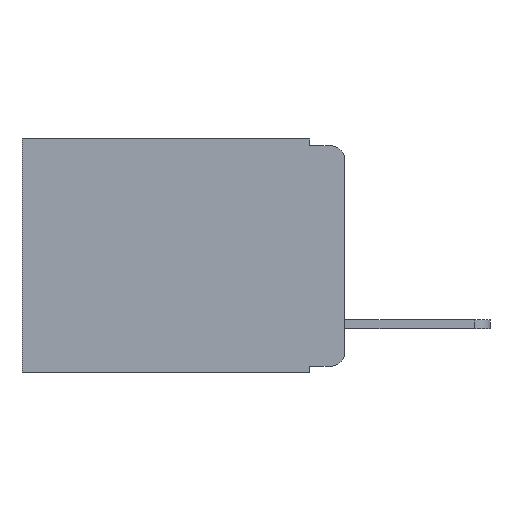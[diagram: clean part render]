
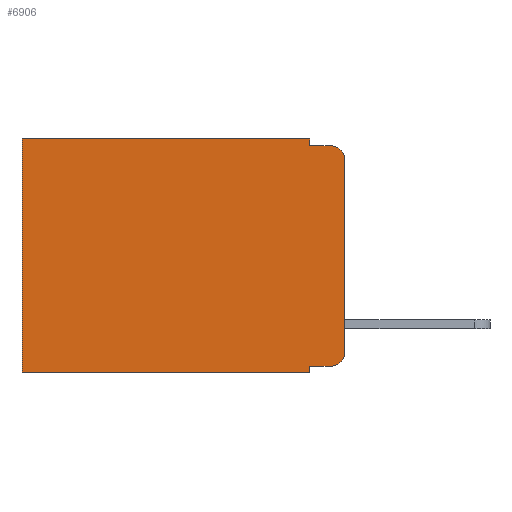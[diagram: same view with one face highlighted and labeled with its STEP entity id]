
A CAD part, left-side view. The second image highlights one B-rep face of the part: STEP entity #6906.
In plain terms, the highlighted planar face has unit normal (-1, 0, 0).
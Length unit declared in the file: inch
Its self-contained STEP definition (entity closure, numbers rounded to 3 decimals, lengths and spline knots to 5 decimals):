
#186 = DIRECTION ( 'NONE',  ( -1., 0., 0. ) ) ;
#322 = VERTEX_POINT ( 'NONE', #6644 ) ;
#1063 = ORIENTED_EDGE ( 'NONE', *, *, #12610, .F. ) ;
#1539 = ORIENTED_EDGE ( 'NONE', *, *, #17304, .T. ) ;
#1707 = PLANE ( 'NONE',  #15708 ) ;
#1716 = AXIS2_PLACEMENT_3D ( 'NONE', #11540, #2862, #12925 ) ;
#1764 = CARTESIAN_POINT ( 'NONE',  ( 0.298, 0.051, -0.333 ) ) ;
#1904 = VERTEX_POINT ( 'NONE', #14746 ) ;
#2031 = ORIENTED_EDGE ( 'NONE', *, *, #14384, .F. ) ;
#2276 = VERTEX_POINT ( 'NONE', #9889 ) ;
#2442 = CARTESIAN_POINT ( 'NONE',  ( 0.298, 0.02, -0.01 ) ) ;
#2471 = ORIENTED_EDGE ( 'NONE', *, *, #9795, .F. ) ;
#2862 = DIRECTION ( 'NONE',  ( -1., 0., 0. ) ) ;
#3031 = DIRECTION ( 'NONE',  ( 0., 1., 0. ) ) ;
#3351 = CARTESIAN_POINT ( 'NONE',  ( 0.298, 0.02, -0.333 ) ) ;
#3567 = EDGE_CURVE ( 'NONE', #14981, #322, #12521, .T. ) ;
#3623 = ORIENTED_EDGE ( 'NONE', *, *, #11748, .F. ) ;
#4083 = CARTESIAN_POINT ( 'NONE',  ( 0.298, 0.051, 0. ) ) ;
#4109 = ORIENTED_EDGE ( 'NONE', *, *, #16272, .T. ) ;
#4199 = LINE ( 'NONE', #12186, #15170 ) ;
#4616 = LINE ( 'NONE', #12272, #8509 ) ;
#4727 = AXIS2_PLACEMENT_3D ( 'NONE', #9014, #186, #10432 ) ;
#5464 = EDGE_CURVE ( 'NONE', #13408, #322, #7833, .T. ) ;
#5963 = EDGE_CURVE ( 'NONE', #9986, #2276, #11130, .T. ) ;
#5988 = CARTESIAN_POINT ( 'NONE',  ( 0.298, 0., -0.03 ) ) ;
#6644 = CARTESIAN_POINT ( 'NONE',  ( 0.298, 0., -0.313 ) ) ;
#6906 = ADVANCED_FACE ( 'NONE', ( #13041 ), #1707, .F. ) ;
#7362 = ORIENTED_EDGE ( 'NONE', *, *, #5464, .T. ) ;
#7469 = CARTESIAN_POINT ( 'NONE',  ( 0.298, 0.051, 0. ) ) ;
#7648 = CARTESIAN_POINT ( 'NONE',  ( 0.298, 0., 0. ) ) ;
#7833 = CIRCLE ( 'NONE', #1716, 0.02 ) ;
#8217 = VERTEX_POINT ( 'NONE', #1764 ) ;
#8253 = LINE ( 'NONE', #7469, #11129 ) ;
#8509 = VECTOR ( 'NONE', #13670, 39.37008 ) ;
#8649 = ORIENTED_EDGE ( 'NONE', *, *, #3567, .F. ) ;
#9014 = CARTESIAN_POINT ( 'NONE',  ( 0.298, 0.02, -0.03 ) ) ;
#9064 = DIRECTION ( 'NONE',  ( 0., 0., -1. ) ) ;
#9400 = LINE ( 'NONE', #12596, #16417 ) ;
#9449 = LINE ( 'NONE', #13087, #17327 ) ;
#9788 = CARTESIAN_POINT ( 'NONE',  ( 0.298, 0.473, 0. ) ) ;
#9795 = EDGE_CURVE ( 'NONE', #15896, #11441, #17621, .T. ) ;
#9889 = CARTESIAN_POINT ( 'NONE',  ( 0.298, 0.473, -0.343 ) ) ;
#9986 = VERTEX_POINT ( 'NONE', #15990 ) ;
#10327 = VERTEX_POINT ( 'NONE', #2442 ) ;
#10432 = DIRECTION ( 'NONE',  ( 0., 0., -1. ) ) ;
#10884 = ORIENTED_EDGE ( 'NONE', *, *, #13651, .T. ) ;
#11129 = VECTOR ( 'NONE', #17346, 39.37008 ) ;
#11130 = LINE ( 'NONE', #9788, #11574 ) ;
#11441 = VERTEX_POINT ( 'NONE', #15159 ) ;
#11540 = CARTESIAN_POINT ( 'NONE',  ( 0.298, 0.02, -0.313 ) ) ;
#11574 = VECTOR ( 'NONE', #14005, 39.37008 ) ;
#11748 = EDGE_CURVE ( 'NONE', #1904, #2276, #9449, .T. ) ;
#12084 = VECTOR ( 'NONE', #18532, 39.37008 ) ;
#12186 = CARTESIAN_POINT ( 'NONE',  ( 0.298, 0.051, -0.333 ) ) ;
#12272 = CARTESIAN_POINT ( 'NONE',  ( 0.298, 0.051, -0.01 ) ) ;
#12521 = LINE ( 'NONE', #18476, #12084 ) ;
#12596 = CARTESIAN_POINT ( 'NONE',  ( 0.298, 0., 0. ) ) ;
#12610 = EDGE_CURVE ( 'NONE', #11441, #10327, #4616, .T. ) ;
#12925 = DIRECTION ( 'NONE',  ( 0., 0., -1. ) ) ;
#13041 = FACE_OUTER_BOUND ( 'NONE', #17484, .T. ) ;
#13087 = CARTESIAN_POINT ( 'NONE',  ( 0.298, 0., -0.343 ) ) ;
#13408 = VERTEX_POINT ( 'NONE', #3351 ) ;
#13456 = VECTOR ( 'NONE', #16752, 39.37008 ) ;
#13590 = DIRECTION ( 'NONE',  ( 0., -1., 0. ) ) ;
#13651 = EDGE_CURVE ( 'NONE', #15896, #9986, #9400, .T. ) ;
#13670 = DIRECTION ( 'NONE',  ( 0., -1., 0. ) ) ;
#13994 = DIRECTION ( 'NONE',  ( 0., 1., 0. ) ) ;
#14005 = DIRECTION ( 'NONE',  ( 0., 0., -1. ) ) ;
#14384 = EDGE_CURVE ( 'NONE', #8217, #1904, #8253, .T. ) ;
#14746 = CARTESIAN_POINT ( 'NONE',  ( 0.298, 0.051, -0.343 ) ) ;
#14981 = VERTEX_POINT ( 'NONE', #5988 ) ;
#15159 = CARTESIAN_POINT ( 'NONE',  ( 0.298, 0.051, -0.01 ) ) ;
#15170 = VECTOR ( 'NONE', #13590, 39.37008 ) ;
#15365 = CARTESIAN_POINT ( 'NONE',  ( 0.298, 0.051, 0. ) ) ;
#15708 = AXIS2_PLACEMENT_3D ( 'NONE', #7648, #17460, #9064 ) ;
#15810 = CIRCLE ( 'NONE', #4727, 0.02 ) ;
#15896 = VERTEX_POINT ( 'NONE', #4083 ) ;
#15990 = CARTESIAN_POINT ( 'NONE',  ( 0.298, 0.473, 0. ) ) ;
#16272 = EDGE_CURVE ( 'NONE', #8217, #13408, #4199, .T. ) ;
#16417 = VECTOR ( 'NONE', #13994, 39.37008 ) ;
#16752 = DIRECTION ( 'NONE',  ( 0., 0., -1. ) ) ;
#17304 = EDGE_CURVE ( 'NONE', #14981, #10327, #15810, .T. ) ;
#17327 = VECTOR ( 'NONE', #3031, 39.37008 ) ;
#17346 = DIRECTION ( 'NONE',  ( 0., 0., -1. ) ) ;
#17446 = ORIENTED_EDGE ( 'NONE', *, *, #5963, .T. ) ;
#17460 = DIRECTION ( 'NONE',  ( 1., 0., 0. ) ) ;
#17484 = EDGE_LOOP ( 'NONE', ( #8649, #1539, #1063, #2471, #10884, #17446, #3623, #2031, #4109, #7362 ) ) ;
#17621 = LINE ( 'NONE', #15365, #13456 ) ;
#18476 = CARTESIAN_POINT ( 'NONE',  ( 0.298, 0., 0. ) ) ;
#18532 = DIRECTION ( 'NONE',  ( 0., 0., -1. ) ) ;
